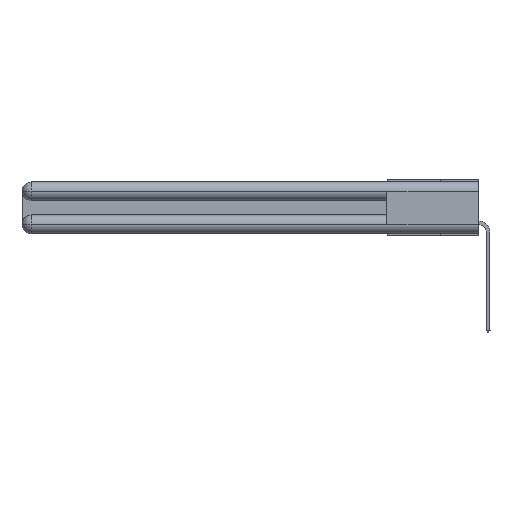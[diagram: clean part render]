
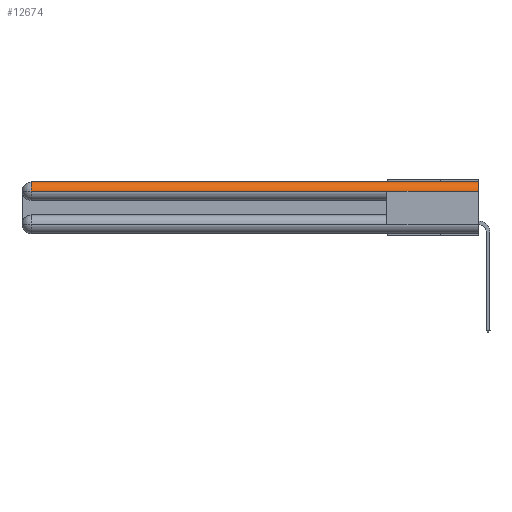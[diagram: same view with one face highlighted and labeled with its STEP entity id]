
A CAD part, left-side view. The second image highlights one B-rep face of the part: STEP entity #12674.
In plain terms, the highlighted cylindrical face has radius 1.562 mm (diameter 3.124 mm), a partial arc.
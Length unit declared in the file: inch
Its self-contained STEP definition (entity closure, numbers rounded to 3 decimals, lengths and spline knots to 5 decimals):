
#69 = CARTESIAN_POINT ( 'NONE',  ( 0.0615, 0., 0. ) ) ;
#1051 = FACE_OUTER_BOUND ( 'NONE', #12154, .T. ) ;
#1184 = CARTESIAN_POINT ( 'NONE',  ( 0.0615, 0., 0. ) ) ;
#2442 = DIRECTION ( 'NONE',  ( 0., -1., 0. ) ) ;
#3149 = DIRECTION ( 'NONE',  ( 0., -1., 0. ) ) ;
#3504 = EDGE_CURVE ( 'NONE', #8662, #28864, #12619, .T. ) ;
#3528 = AXIS2_PLACEMENT_3D ( 'NONE', #22279, #29773, #29880 ) ;
#3942 = LINE ( 'NONE', #25743, #12500 ) ;
#4033 = VECTOR ( 'NONE', #2442, 39.37008 ) ;
#5244 = EDGE_CURVE ( 'NONE', #28864, #21268, #3942, .T. ) ;
#5273 = AXIS2_PLACEMENT_3D ( 'NONE', #7752, #3149, #7862 ) ;
#5647 = CARTESIAN_POINT ( 'NONE',  ( 0.0615, 2.94, 0. ) ) ;
#6123 = ORIENTED_EDGE ( 'NONE', *, *, #23759, .F. ) ;
#7389 = CIRCLE ( 'NONE', #5273, 0.0615 ) ;
#7752 = CARTESIAN_POINT ( 'NONE',  ( 0.0615, 0., -0.0615 ) ) ;
#7800 = AXIS2_PLACEMENT_3D ( 'NONE', #22820, #30339, #16143 ) ;
#7862 = DIRECTION ( 'NONE',  ( 1., 0., 0. ) ) ;
#8662 = VERTEX_POINT ( 'NONE', #5647 ) ;
#8808 = VERTEX_POINT ( 'NONE', #1184 ) ;
#9777 = EDGE_CURVE ( 'NONE', #8808, #25403, #7389, .T. ) ;
#9993 = ORIENTED_EDGE ( 'NONE', *, *, #10166, .F. ) ;
#10166 = EDGE_CURVE ( 'NONE', #25403, #21268, #10358, .T. ) ;
#10358 = LINE ( 'NONE', #24772, #21164 ) ;
#12154 = EDGE_LOOP ( 'NONE', ( #6123, #12777, #16536, #9993, #25343 ) ) ;
#12500 = VECTOR ( 'NONE', #28559, 39.37008 ) ;
#12619 = CIRCLE ( 'NONE', #7800, 0.0615 ) ;
#12674 = ADVANCED_FACE ( 'NONE', ( #1051 ), #19305, .T. ) ;
#12777 = ORIENTED_EDGE ( 'NONE', *, *, #3504, .T. ) ;
#14955 = DIRECTION ( 'NONE',  ( 0., 1., 0. ) ) ;
#16092 = CARTESIAN_POINT ( 'NONE',  ( 0., 0., -0.0615 ) ) ;
#16143 = DIRECTION ( 'NONE',  ( 0., 0., 1. ) ) ;
#16536 = ORIENTED_EDGE ( 'NONE', *, *, #5244, .T. ) ;
#16720 = CARTESIAN_POINT ( 'NONE',  ( 0., 0.6, -0.0615 ) ) ;
#19305 = CYLINDRICAL_SURFACE ( 'NONE', #3528, 0.0615 ) ;
#21164 = VECTOR ( 'NONE', #14955, 39.37008 ) ;
#21217 = CARTESIAN_POINT ( 'NONE',  ( 0., 2.94, -0.0615 ) ) ;
#21268 = VERTEX_POINT ( 'NONE', #16720 ) ;
#22279 = CARTESIAN_POINT ( 'NONE',  ( 0.0615, 0., -0.0615 ) ) ;
#22820 = CARTESIAN_POINT ( 'NONE',  ( 0.0615, 2.94, -0.0615 ) ) ;
#23759 = EDGE_CURVE ( 'NONE', #8662, #8808, #28292, .T. ) ;
#24772 = CARTESIAN_POINT ( 'NONE',  ( 0., 3., -0.0615 ) ) ;
#25343 = ORIENTED_EDGE ( 'NONE', *, *, #9777, .F. ) ;
#25403 = VERTEX_POINT ( 'NONE', #16092 ) ;
#25743 = CARTESIAN_POINT ( 'NONE',  ( 0., 3., -0.0615 ) ) ;
#28292 = LINE ( 'NONE', #69, #4033 ) ;
#28559 = DIRECTION ( 'NONE',  ( 0., -1., 0. ) ) ;
#28864 = VERTEX_POINT ( 'NONE', #21217 ) ;
#29773 = DIRECTION ( 'NONE',  ( 0., 1., 0. ) ) ;
#29880 = DIRECTION ( 'NONE',  ( 0., 0., 1. ) ) ;
#30339 = DIRECTION ( 'NONE',  ( 0., -1., 0. ) ) ;
